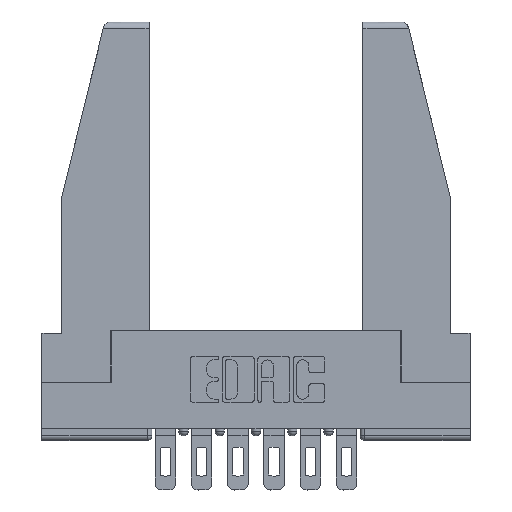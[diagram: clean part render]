
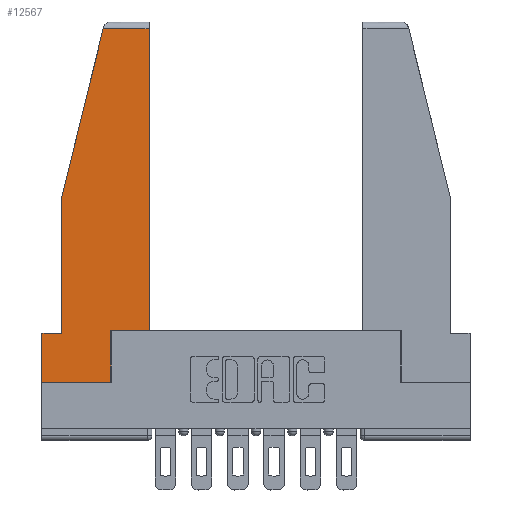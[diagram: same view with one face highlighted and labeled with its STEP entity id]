
A CAD part, top view. The second image highlights one B-rep face of the part: STEP entity #12567.
In plain terms, the highlighted planar face has unit normal (0, 0, 1).
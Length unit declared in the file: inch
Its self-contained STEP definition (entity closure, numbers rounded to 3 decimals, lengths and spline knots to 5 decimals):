
#92 = CARTESIAN_POINT ( 'NONE',  ( 0.2636, 1.52, 0. ) ) ;
#97 = EDGE_CURVE ( 'NONE', #12619, #2603, #10552, .T. ) ;
#209 = CARTESIAN_POINT ( 'NONE',  ( 0., 0.21, 0. ) ) ;
#355 = DIRECTION ( 'NONE',  ( -0.239, -0.971, 0. ) ) ;
#680 = ORIENTED_EDGE ( 'NONE', *, *, #97, .T. ) ;
#703 = CARTESIAN_POINT ( 'NONE',  ( 0.086, 0.21, 0. ) ) ;
#938 = CARTESIAN_POINT ( 'NONE',  ( 0., 0., 0. ) ) ;
#971 = EDGE_LOOP ( 'NONE', ( #2049, #12811, #7328, #2649, #1253, #9065, #8790, #5457, #680 ) ) ;
#1006 = DIRECTION ( 'NONE',  ( 0., 0., 1. ) ) ;
#1083 = LINE ( 'NONE', #10065, #11559 ) ;
#1127 = FACE_OUTER_BOUND ( 'NONE', #971, .T. ) ;
#1253 = ORIENTED_EDGE ( 'NONE', *, *, #2388, .T. ) ;
#1469 = CARTESIAN_POINT ( 'NONE',  ( 0., 0., 0. ) ) ;
#1484 = CARTESIAN_POINT ( 'NONE',  ( 0., 1.52, 0. ) ) ;
#1609 = DIRECTION ( 'NONE',  ( 1., 0., 0. ) ) ;
#1891 = EDGE_CURVE ( 'NONE', #4080, #8316, #11493, .T. ) ;
#2049 = ORIENTED_EDGE ( 'NONE', *, *, #2595, .T. ) ;
#2388 = EDGE_CURVE ( 'NONE', #6621, #3433, #10708, .T. ) ;
#2536 = LINE ( 'NONE', #10377, #6454 ) ;
#2595 = EDGE_CURVE ( 'NONE', #2603, #4707, #11930, .T. ) ;
#2603 = VERTEX_POINT ( 'NONE', #3169 ) ;
#2649 = ORIENTED_EDGE ( 'NONE', *, *, #5329, .T. ) ;
#2666 = EDGE_CURVE ( 'NONE', #9834, #9637, #2536, .T. ) ;
#2869 = CARTESIAN_POINT ( 'NONE',  ( 0.086, 0.8, 0. ) ) ;
#3169 = CARTESIAN_POINT ( 'NONE',  ( 0.461, 0.223, 0. ) ) ;
#3354 = LINE ( 'NONE', #1484, #7408 ) ;
#3433 = VERTEX_POINT ( 'NONE', #209 ) ;
#4080 = VERTEX_POINT ( 'NONE', #10460 ) ;
#4094 = CARTESIAN_POINT ( 'NONE',  ( 0.461, 1.52, 0. ) ) ;
#4707 = VERTEX_POINT ( 'NONE', #4094 ) ;
#4780 = DIRECTION ( 'NONE',  ( 0., -1., 0. ) ) ;
#5329 = EDGE_CURVE ( 'NONE', #9637, #6621, #6885, .T. ) ;
#5334 = AXIS2_PLACEMENT_3D ( 'NONE', #938, #1006, #11933 ) ;
#5397 = VECTOR ( 'NONE', #4780, 39.37008 ) ;
#5457 = ORIENTED_EDGE ( 'NONE', *, *, #12171, .T. ) ;
#5597 = VECTOR ( 'NONE', #6747, 39.37008 ) ;
#5776 = CARTESIAN_POINT ( 'NONE',  ( 0., 0.21, 0. ) ) ;
#5983 = DIRECTION ( 'NONE',  ( 0., 1., 0. ) ) ;
#6454 = VECTOR ( 'NONE', #355, 39.37008 ) ;
#6581 = CARTESIAN_POINT ( 'NONE',  ( 0.297, 0.223, 0. ) ) ;
#6621 = VERTEX_POINT ( 'NONE', #703 ) ;
#6734 = CARTESIAN_POINT ( 'NONE',  ( 0.086, 0.8, 0. ) ) ;
#6747 = DIRECTION ( 'NONE',  ( -1., 0., 0. ) ) ;
#6885 = LINE ( 'NONE', #2869, #5397 ) ;
#6938 = CARTESIAN_POINT ( 'NONE',  ( 0.461, 0.223, 0. ) ) ;
#7066 = CARTESIAN_POINT ( 'NONE',  ( 0.297, 0.223, 0. ) ) ;
#7328 = ORIENTED_EDGE ( 'NONE', *, *, #2666, .T. ) ;
#7408 = VECTOR ( 'NONE', #10486, 39.37008 ) ;
#7457 = EDGE_CURVE ( 'NONE', #3433, #4080, #9811, .T. ) ;
#7721 = CARTESIAN_POINT ( 'NONE',  ( 0., 0.21, 0. ) ) ;
#7853 = PLANE ( 'NONE',  #5334 ) ;
#7923 = DIRECTION ( 'NONE',  ( 0., -1., 0. ) ) ;
#8316 = VERTEX_POINT ( 'NONE', #10626 ) ;
#8790 = ORIENTED_EDGE ( 'NONE', *, *, #1891, .T. ) ;
#9009 = DIRECTION ( 'NONE',  ( 0., 1., 0. ) ) ;
#9065 = ORIENTED_EDGE ( 'NONE', *, *, #7457, .T. ) ;
#9553 = DIRECTION ( 'NONE',  ( 1., 0., 0. ) ) ;
#9637 = VERTEX_POINT ( 'NONE', #6734 ) ;
#9657 = VECTOR ( 'NONE', #9553, 39.37008 ) ;
#9762 = VECTOR ( 'NONE', #1609, 39.37008 ) ;
#9811 = LINE ( 'NONE', #5776, #12132 ) ;
#9834 = VERTEX_POINT ( 'NONE', #92 ) ;
#10065 = CARTESIAN_POINT ( 'NONE',  ( 0.297, 0., 0. ) ) ;
#10377 = CARTESIAN_POINT ( 'NONE',  ( 0.271, 1.55, 0. ) ) ;
#10460 = CARTESIAN_POINT ( 'NONE',  ( 0., 0., 0. ) ) ;
#10486 = DIRECTION ( 'NONE',  ( -1., 0., 0. ) ) ;
#10552 = LINE ( 'NONE', #6581, #9762 ) ;
#10626 = CARTESIAN_POINT ( 'NONE',  ( 0.297, 0., 0. ) ) ;
#10708 = LINE ( 'NONE', #7721, #5597 ) ;
#11467 = EDGE_CURVE ( 'NONE', #4707, #9834, #3354, .T. ) ;
#11493 = LINE ( 'NONE', #1469, #9657 ) ;
#11559 = VECTOR ( 'NONE', #5983, 39.37008 ) ;
#11930 = LINE ( 'NONE', #6938, #12696 ) ;
#11933 = DIRECTION ( 'NONE',  ( 1., 0., 0. ) ) ;
#12132 = VECTOR ( 'NONE', #7923, 39.37008 ) ;
#12171 = EDGE_CURVE ( 'NONE', #8316, #12619, #1083, .T. ) ;
#12567 = ADVANCED_FACE ( 'NONE', ( #1127 ), #7853, .T. ) ;
#12619 = VERTEX_POINT ( 'NONE', #7066 ) ;
#12696 = VECTOR ( 'NONE', #9009, 39.37008 ) ;
#12811 = ORIENTED_EDGE ( 'NONE', *, *, #11467, .T. ) ;
